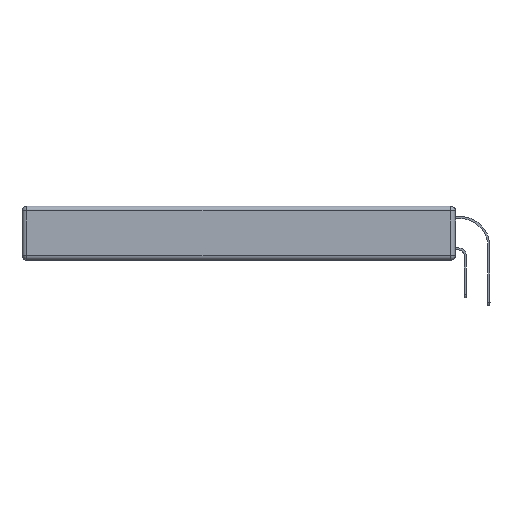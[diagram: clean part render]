
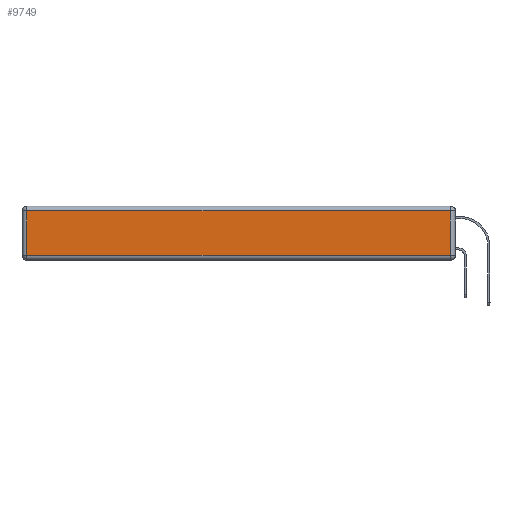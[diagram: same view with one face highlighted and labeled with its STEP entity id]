
A CAD part, left-side view. The second image highlights one B-rep face of the part: STEP entity #9749.
In plain terms, the highlighted planar face has unit normal (-1, 0, 0).
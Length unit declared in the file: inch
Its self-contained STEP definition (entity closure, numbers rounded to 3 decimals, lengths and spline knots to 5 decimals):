
#857 = DIRECTION ( 'NONE',  ( 0., 0., 1. ) ) ;
#1001 = AXIS2_PLACEMENT_3D ( 'NONE', #3369, #13725, #857 ) ;
#2794 = DIRECTION ( 'NONE',  ( 0., 0., 1. ) ) ;
#2965 = CARTESIAN_POINT ( 'NONE',  ( 0., 2.72, -0.313 ) ) ;
#3030 = EDGE_CURVE ( 'NONE', #6996, #5590, #3450, .T. ) ;
#3297 = ORIENTED_EDGE ( 'NONE', *, *, #3030, .T. ) ;
#3369 = CARTESIAN_POINT ( 'NONE',  ( 0., 0., -0.343 ) ) ;
#3450 = LINE ( 'NONE', #8833, #13673 ) ;
#4570 = FACE_OUTER_BOUND ( 'NONE', #14810, .T. ) ;
#4770 = VERTEX_POINT ( 'NONE', #2965 ) ;
#5452 = LINE ( 'NONE', #15556, #12033 ) ;
#5590 = VERTEX_POINT ( 'NONE', #10933 ) ;
#6053 = DIRECTION ( 'NONE',  ( 0., 1., 0. ) ) ;
#6597 = VERTEX_POINT ( 'NONE', #13896 ) ;
#6996 = VERTEX_POINT ( 'NONE', #9233 ) ;
#8348 = EDGE_CURVE ( 'NONE', #5590, #4770, #9767, .T. ) ;
#8703 = CARTESIAN_POINT ( 'NONE',  ( 0., 2.72, -0.343 ) ) ;
#8833 = CARTESIAN_POINT ( 'NONE',  ( 0., 2.75, -0.03 ) ) ;
#9007 = EDGE_CURVE ( 'NONE', #6597, #6996, #5452, .T. ) ;
#9217 = EDGE_CURVE ( 'NONE', #4770, #6597, #11491, .T. ) ;
#9233 = CARTESIAN_POINT ( 'NONE',  ( 0., 0.03, -0.03 ) ) ;
#9355 = ORIENTED_EDGE ( 'NONE', *, *, #9217, .T. ) ;
#9749 = ADVANCED_FACE ( 'NONE', ( #4570 ), #12687, .T. ) ;
#9767 = LINE ( 'NONE', #8703, #12003 ) ;
#10933 = CARTESIAN_POINT ( 'NONE',  ( 0., 2.72, -0.03 ) ) ;
#11017 = ORIENTED_EDGE ( 'NONE', *, *, #8348, .T. ) ;
#11066 = DIRECTION ( 'NONE',  ( 0., 0., -1. ) ) ;
#11491 = LINE ( 'NONE', #16516, #16990 ) ;
#12003 = VECTOR ( 'NONE', #11066, 39.37008 ) ;
#12033 = VECTOR ( 'NONE', #2794, 39.37008 ) ;
#12546 = ORIENTED_EDGE ( 'NONE', *, *, #9007, .T. ) ;
#12687 = PLANE ( 'NONE',  #1001 ) ;
#13673 = VECTOR ( 'NONE', #6053, 39.37008 ) ;
#13725 = DIRECTION ( 'NONE',  ( -1., 0., 0. ) ) ;
#13896 = CARTESIAN_POINT ( 'NONE',  ( 0., 0.03, -0.313 ) ) ;
#13986 = DIRECTION ( 'NONE',  ( 0., -1., 0. ) ) ;
#14810 = EDGE_LOOP ( 'NONE', ( #9355, #12546, #3297, #11017 ) ) ;
#15556 = CARTESIAN_POINT ( 'NONE',  ( 0., 0.03, -0.343 ) ) ;
#16516 = CARTESIAN_POINT ( 'NONE',  ( 0., 0., -0.313 ) ) ;
#16990 = VECTOR ( 'NONE', #13986, 39.37008 ) ;
